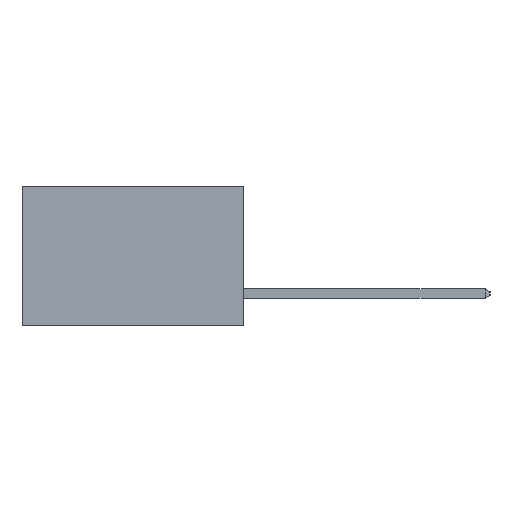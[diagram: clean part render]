
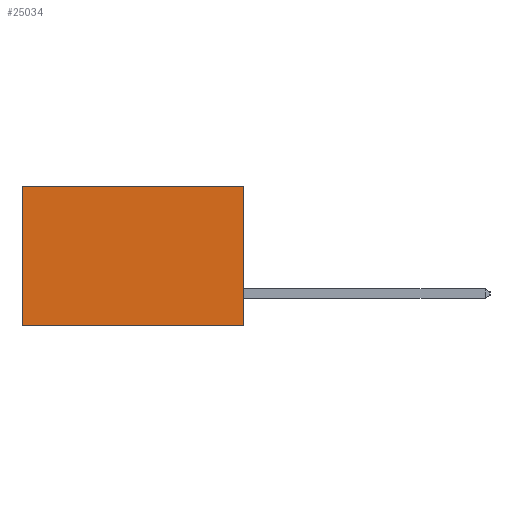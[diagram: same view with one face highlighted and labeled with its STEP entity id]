
A CAD part, left-side view. The second image highlights one B-rep face of the part: STEP entity #25034.
In plain terms, the highlighted planar face has unit normal (-1, 0, 0).
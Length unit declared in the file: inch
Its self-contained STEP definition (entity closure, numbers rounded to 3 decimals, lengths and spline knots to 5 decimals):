
#1002 = LINE ( 'NONE', #29142, #7095 ) ;
#2793 = LINE ( 'NONE', #15562, #7450 ) ;
#4971 = CARTESIAN_POINT ( 'NONE',  ( 0.277, 0.59, -0.37 ) ) ;
#5074 = VERTEX_POINT ( 'NONE', #15479 ) ;
#6419 = VECTOR ( 'NONE', #19914, 39.37008 ) ;
#7076 = EDGE_CURVE ( 'NONE', #21020, #5074, #2793, .T. ) ;
#7095 = VECTOR ( 'NONE', #11380, 39.37008 ) ;
#7450 = VECTOR ( 'NONE', #15934, 39.37008 ) ;
#9854 = ORIENTED_EDGE ( 'NONE', *, *, #7076, .T. ) ;
#9955 = DIRECTION ( 'NONE',  ( 0., 0., -1. ) ) ;
#11380 = DIRECTION ( 'NONE',  ( 0., 0., -1. ) ) ;
#12410 = DIRECTION ( 'NONE',  ( 0., 1., 0. ) ) ;
#13125 = CARTESIAN_POINT ( 'NONE',  ( 0.277, 0.59, -0.37 ) ) ;
#14444 = CARTESIAN_POINT ( 'NONE',  ( 0.277, 0., -0.37 ) ) ;
#15149 = VECTOR ( 'NONE', #12410, 39.37008 ) ;
#15479 = CARTESIAN_POINT ( 'NONE',  ( 0.277, 0.59, 0. ) ) ;
#15562 = CARTESIAN_POINT ( 'NONE',  ( 0.277, 0., 0. ) ) ;
#15934 = DIRECTION ( 'NONE',  ( 0., 1., 0. ) ) ;
#18244 = EDGE_CURVE ( 'NONE', #27188, #25572, #26233, .T. ) ;
#19914 = DIRECTION ( 'NONE',  ( 0., 0., -1. ) ) ;
#19978 = EDGE_LOOP ( 'NONE', ( #24236, #25612, #26297, #9854 ) ) ;
#20058 = CARTESIAN_POINT ( 'NONE',  ( 0.277, 0., 0. ) ) ;
#20288 = FACE_OUTER_BOUND ( 'NONE', #19978, .T. ) ;
#21020 = VERTEX_POINT ( 'NONE', #20058 ) ;
#21189 = PLANE ( 'NONE',  #27868 ) ;
#21469 = CARTESIAN_POINT ( 'NONE',  ( 0.277, 0., -0.37 ) ) ;
#23411 = DIRECTION ( 'NONE',  ( 1., 0., 0. ) ) ;
#24236 = ORIENTED_EDGE ( 'NONE', *, *, #25312, .T. ) ;
#24414 = LINE ( 'NONE', #13125, #6419 ) ;
#25034 = ADVANCED_FACE ( 'NONE', ( #20288 ), #21189, .F. ) ;
#25312 = EDGE_CURVE ( 'NONE', #5074, #25572, #24414, .T. ) ;
#25572 = VERTEX_POINT ( 'NONE', #4971 ) ;
#25612 = ORIENTED_EDGE ( 'NONE', *, *, #18244, .F. ) ;
#26233 = LINE ( 'NONE', #21469, #15149 ) ;
#26297 = ORIENTED_EDGE ( 'NONE', *, *, #29054, .F. ) ;
#26631 = CARTESIAN_POINT ( 'NONE',  ( 0.277, 0., -0.37 ) ) ;
#27188 = VERTEX_POINT ( 'NONE', #26631 ) ;
#27868 = AXIS2_PLACEMENT_3D ( 'NONE', #14444, #23411, #9955 ) ;
#29054 = EDGE_CURVE ( 'NONE', #21020, #27188, #1002, .T. ) ;
#29142 = CARTESIAN_POINT ( 'NONE',  ( 0.277, 0., -0.37 ) ) ;
